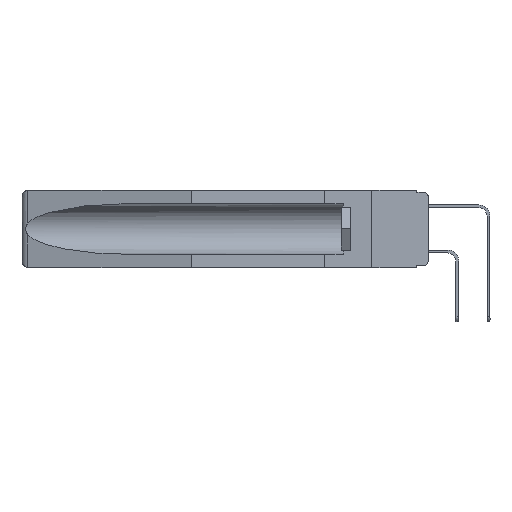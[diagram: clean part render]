
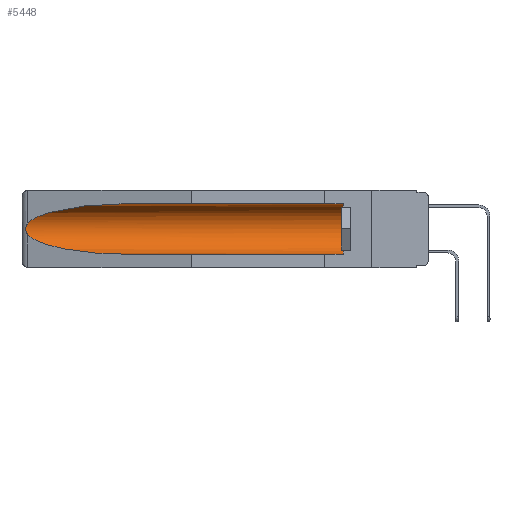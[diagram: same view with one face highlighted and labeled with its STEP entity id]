
A CAD part, left-side view. The second image highlights one B-rep face of the part: STEP entity #5448.
In plain terms, the highlighted cylindrical face has radius 2.857 mm (diameter 5.715 mm), a partial arc.
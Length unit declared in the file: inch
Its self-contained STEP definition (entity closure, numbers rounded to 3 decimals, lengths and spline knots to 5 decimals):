
#138 = CARTESIAN_POINT ( 'NONE',  ( 0.21114, 1.30732, -0.284 ) ) ;
#198 = CARTESIAN_POINT ( 'NONE',  ( 0.155, -0.30754, -0.284 ) ) ;
#579 = DIRECTION ( 'NONE',  ( 0., 0., 1. ) ) ;
#745 = DIRECTION ( 'NONE',  ( 0., 0., 1. ) ) ;
#842 = ORIENTED_EDGE ( 'NONE', *, *, #9425, .F. ) ;
#1308 = CARTESIAN_POINT ( 'NONE',  ( 0.155, 0.126, -0.059 ) ) ;
#1620 = CARTESIAN_POINT ( 'NONE',  ( 0.25451, 1.48313, -0.24835 ) ) ;
#1798 = EDGE_CURVE ( 'NONE', #16725, #8814, #8134, .T. ) ;
#2009 = VERTEX_POINT ( 'NONE', #12335 ) ;
#2069 = EDGE_CURVE ( 'NONE', #2009, #7615, #17675, .T. ) ;
#2253 = DIRECTION ( 'NONE',  ( 0., 1., 0. ) ) ;
#3703 = CARTESIAN_POINT ( 'NONE',  ( 0.26537, 1.52718, -0.19328 ) ) ;
#4190 = LINE ( 'NONE', #198, #8624 ) ;
#4253 = ORIENTED_EDGE ( 'NONE', *, *, #1798, .T. ) ;
#5078 = CARTESIAN_POINT ( 'NONE',  ( 0.26537, 1.52718, -0.14972 ) ) ;
#5261 = CARTESIAN_POINT ( 'NONE',  ( 0.2673, 1.5327, -0.16383 ) ) ;
#5448 = ADVANCED_FACE ( 'NONE', ( #14552 ), #16120, .F. ) ;
#5697 = CARTESIAN_POINT ( 'NONE',  ( 0.26537, 1.52718, -0.19328 ) ) ;
#5839 = CARTESIAN_POINT ( 'NONE',  ( 0.26537, 1.52718, -0.14972 ) ) ;
#6313 = DIRECTION ( 'NONE',  ( 0., -1., 0. ) ) ;
#6716 = B_SPLINE_CURVE_WITH_KNOTS ( 'NONE', 3,
 ( #5078, #15246, #10713, #5261, #6741, #8045, #9432, #10808, #15061, #3703 ),
 .UNSPECIFIED., .F., .F.,
 ( 4, 2, 2, 2, 4 ),
 ( 0., 0.00029, 0.00058, 0.00087, 0.00117 ),
 .UNSPECIFIED. ) ;
#6741 = CARTESIAN_POINT ( 'NONE',  ( 0.2675, 1.53308, -0.16763 ) ) ;
#7353 = EDGE_CURVE ( 'NONE', #13006, #9337, #13918, .T. ) ;
#7615 = VERTEX_POINT ( 'NONE', #5839 ) ;
#7914 = DIRECTION ( 'NONE',  ( 0., 1., 0. ) ) ;
#8045 = CARTESIAN_POINT ( 'NONE',  ( 0.2675, 1.53308, -0.17534 ) ) ;
#8134 =( BOUNDED_CURVE ( )  B_SPLINE_CURVE ( 3, ( #5697, #1620, #138, #12625 ),
 .UNSPECIFIED., .F., .F. ) 
 B_SPLINE_CURVE_WITH_KNOTS ( ( 4, 4 ),
 ( 0.1948, 1.5708 ),
 .UNSPECIFIED. ) 
 CURVE ( )  GEOMETRIC_REPRESENTATION_ITEM ( )  RATIONAL_B_SPLINE_CURVE ( ( 1., 0.848, 0.848, 1. ) ) 
 REPRESENTATION_ITEM ( '' )  );
#8624 = VECTOR ( 'NONE', #16847, 39.37008 ) ;
#8814 = VERTEX_POINT ( 'NONE', #11199 ) ;
#9196 = AXIS2_PLACEMENT_3D ( 'NONE', #16308, #2253, #579 ) ;
#9337 = VERTEX_POINT ( 'NONE', #1308 ) ;
#9383 = CARTESIAN_POINT ( 'NONE',  ( 0.25451, 1.48313, -0.09465 ) ) ;
#9425 = EDGE_CURVE ( 'NONE', #13006, #8814, #4190, .T. ) ;
#9432 = CARTESIAN_POINT ( 'NONE',  ( 0.2673, 1.53269, -0.17917 ) ) ;
#9500 = AXIS2_PLACEMENT_3D ( 'NONE', #13415, #6313, #745 ) ;
#9874 = ORIENTED_EDGE ( 'NONE', *, *, #2069, .T. ) ;
#10204 = CARTESIAN_POINT ( 'NONE',  ( 0.26537, 1.52718, -0.19328 ) ) ;
#10671 = LINE ( 'NONE', #13620, #17813 ) ;
#10713 = CARTESIAN_POINT ( 'NONE',  ( 0.26654, 1.53092, -0.15636 ) ) ;
#10808 = CARTESIAN_POINT ( 'NONE',  ( 0.26655, 1.53094, -0.18657 ) ) ;
#11036 = CARTESIAN_POINT ( 'NONE',  ( 0.21114, 1.30732, -0.059 ) ) ;
#11199 = CARTESIAN_POINT ( 'NONE',  ( 0.155, 1.07973, -0.284 ) ) ;
#11223 = ORIENTED_EDGE ( 'NONE', *, *, #12214, .T. ) ;
#11327 = ORIENTED_EDGE ( 'NONE', *, *, #7353, .T. ) ;
#11522 = EDGE_LOOP ( 'NONE', ( #9874, #14024, #4253, #842, #11327, #11223 ) ) ;
#11662 = CARTESIAN_POINT ( 'NONE',  ( 0.155, 0.126, -0.284 ) ) ;
#12214 = EDGE_CURVE ( 'NONE', #9337, #2009, #10671, .T. ) ;
#12335 = CARTESIAN_POINT ( 'NONE',  ( 0.155, 1.07973, -0.059 ) ) ;
#12625 = CARTESIAN_POINT ( 'NONE',  ( 0.155, 1.07973, -0.284 ) ) ;
#13006 = VERTEX_POINT ( 'NONE', #11662 ) ;
#13415 = CARTESIAN_POINT ( 'NONE',  ( 0.155, 0.126, -0.1715 ) ) ;
#13620 = CARTESIAN_POINT ( 'NONE',  ( 0.155, -0.30754, -0.059 ) ) ;
#13918 = CIRCLE ( 'NONE', #9500, 0.1125 ) ;
#14024 = ORIENTED_EDGE ( 'NONE', *, *, #16167, .T. ) ;
#14552 = FACE_OUTER_BOUND ( 'NONE', #11522, .T. ) ;
#15061 = CARTESIAN_POINT ( 'NONE',  ( 0.26597, 1.5296, -0.19026 ) ) ;
#15246 = CARTESIAN_POINT ( 'NONE',  ( 0.26597, 1.52961, -0.15275 ) ) ;
#16120 = CYLINDRICAL_SURFACE ( 'NONE', #9196, 0.1125 ) ;
#16167 = EDGE_CURVE ( 'NONE', #7615, #16725, #6716, .T. ) ;
#16308 = CARTESIAN_POINT ( 'NONE',  ( 0.155, -0.30754, -0.1715 ) ) ;
#16399 = CARTESIAN_POINT ( 'NONE',  ( 0.155, 1.07973, -0.059 ) ) ;
#16674 = CARTESIAN_POINT ( 'NONE',  ( 0.26537, 1.52718, -0.14972 ) ) ;
#16725 = VERTEX_POINT ( 'NONE', #10204 ) ;
#16847 = DIRECTION ( 'NONE',  ( 0., 1., 0. ) ) ;
#17675 =( BOUNDED_CURVE ( )  B_SPLINE_CURVE ( 3, ( #16399, #11036, #9383, #16674 ),
 .UNSPECIFIED., .F., .F. ) 
 B_SPLINE_CURVE_WITH_KNOTS ( ( 4, 4 ),
 ( 4.71239, 6.08839 ),
 .UNSPECIFIED. ) 
 CURVE ( )  GEOMETRIC_REPRESENTATION_ITEM ( )  RATIONAL_B_SPLINE_CURVE ( ( 1., 0.848, 0.848, 1. ) ) 
 REPRESENTATION_ITEM ( '' )  );
#17813 = VECTOR ( 'NONE', #7914, 39.37008 ) ;
